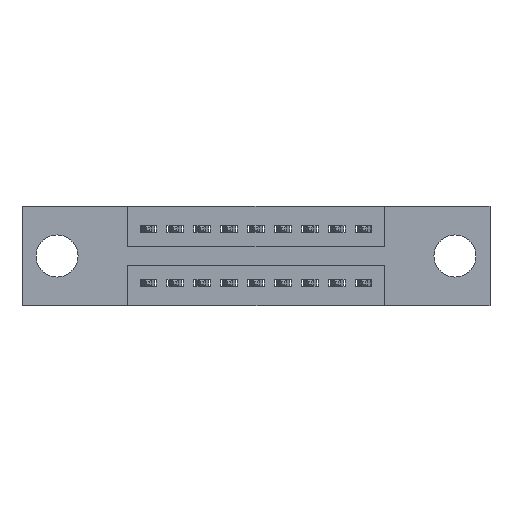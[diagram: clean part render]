
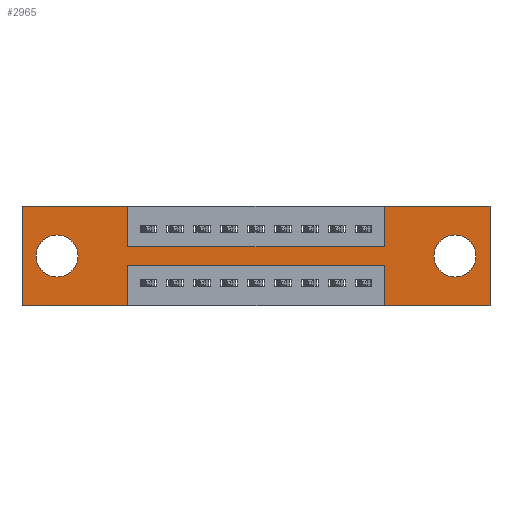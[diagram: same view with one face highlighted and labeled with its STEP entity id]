
A CAD part, front view. The second image highlights one B-rep face of the part: STEP entity #2965.
In plain terms, the highlighted planar face has unit normal (0, -1, 0).
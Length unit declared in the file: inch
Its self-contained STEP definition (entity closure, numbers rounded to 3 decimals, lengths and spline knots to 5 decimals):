
#74 = VERTEX_POINT ( 'NONE', #2329 ) ;
#160 = DIRECTION ( 'NONE',  ( 0., 0., 1. ) ) ;
#163 = VERTEX_POINT ( 'NONE', #8953 ) ;
#263 = DIRECTION ( 'NONE',  ( 0., 1., 0. ) ) ;
#372 = ORIENTED_EDGE ( 'NONE', *, *, #6283, .F. ) ;
#404 = ORIENTED_EDGE ( 'NONE', *, *, #4844, .F. ) ;
#423 = VERTEX_POINT ( 'NONE', #2195 ) ;
#517 = LINE ( 'NONE', #7329, #3308 ) ;
#692 = FACE_BOUND ( 'NONE', #3170, .T. ) ;
#868 = CARTESIAN_POINT ( 'NONE',  ( 0.3925, 0., -0.22 ) ) ;
#878 = PLANE ( 'NONE',  #1869 ) ;
#967 = VERTEX_POINT ( 'NONE', #7991 ) ;
#1048 = DIRECTION ( 'NONE',  ( 0., -1., 0. ) ) ;
#1077 = CARTESIAN_POINT ( 'NONE',  ( 1.3425, 0., 0. ) ) ;
#1246 = LINE ( 'NONE', #7580, #3026 ) ;
#1304 = ORIENTED_EDGE ( 'NONE', *, *, #8334, .T. ) ;
#1322 = ORIENTED_EDGE ( 'NONE', *, *, #5322, .T. ) ;
#1618 = DIRECTION ( 'NONE',  ( 0., 1., 0. ) ) ;
#1650 = ORIENTED_EDGE ( 'NONE', *, *, #9314, .F. ) ;
#1763 = CARTESIAN_POINT ( 'NONE',  ( 1.605, 0., -0.107 ) ) ;
#1867 = ORIENTED_EDGE ( 'NONE', *, *, #5052, .F. ) ;
#1869 = AXIS2_PLACEMENT_3D ( 'NONE', #3627, #1048, #10817 ) ;
#1968 = ORIENTED_EDGE ( 'NONE', *, *, #8434, .F. ) ;
#2028 = EDGE_CURVE ( 'NONE', #74, #2369, #5194, .T. ) ;
#2097 = VECTOR ( 'NONE', #3045, 39.37008 ) ;
#2189 = LINE ( 'NONE', #2750, #8909 ) ;
#2195 = CARTESIAN_POINT ( 'NONE',  ( 0.3925, 0., -0.15 ) ) ;
#2329 = CARTESIAN_POINT ( 'NONE',  ( 1.3425, 0., -0.22 ) ) ;
#2369 = VERTEX_POINT ( 'NONE', #9668 ) ;
#2477 = VERTEX_POINT ( 'NONE', #9061 ) ;
#2519 = VECTOR ( 'NONE', #4711, 39.37008 ) ;
#2556 = EDGE_CURVE ( 'NONE', #2369, #6684, #2641, .T. ) ;
#2635 = CARTESIAN_POINT ( 'NONE',  ( 1.605, 0., -0.185 ) ) ;
#2641 = LINE ( 'NONE', #6640, #2097 ) ;
#2654 = CARTESIAN_POINT ( 'NONE',  ( 0.3925, 0., -0.37 ) ) ;
#2666 = DIRECTION ( 'NONE',  ( 0., 1., 0. ) ) ;
#2750 = CARTESIAN_POINT ( 'NONE',  ( 0., 0., -0.37 ) ) ;
#2965 = ADVANCED_FACE ( 'NONE', ( #8938, #692, #6413 ), #878, .T. ) ;
#2986 = VERTEX_POINT ( 'NONE', #4615 ) ;
#3002 = CARTESIAN_POINT ( 'NONE',  ( 1.735, 0., 0. ) ) ;
#3004 = VECTOR ( 'NONE', #5814, 39.37008 ) ;
#3006 = CARTESIAN_POINT ( 'NONE',  ( 1.605, 0., -0.185 ) ) ;
#3026 = VECTOR ( 'NONE', #6043, 39.37008 ) ;
#3045 = DIRECTION ( 'NONE',  ( 0., 0., -1. ) ) ;
#3170 = EDGE_LOOP ( 'NONE', ( #1304, #4681 ) ) ;
#3264 = CARTESIAN_POINT ( 'NONE',  ( 0.13, 0., -0.185 ) ) ;
#3308 = VECTOR ( 'NONE', #6284, 39.37008 ) ;
#3390 = VECTOR ( 'NONE', #3605, 39.37008 ) ;
#3605 = DIRECTION ( 'NONE',  ( 0., 0., 1. ) ) ;
#3627 = CARTESIAN_POINT ( 'NONE',  ( 0., 0., -0.37 ) ) ;
#3881 = CIRCLE ( 'NONE', #6200, 0.078 ) ;
#4049 = CARTESIAN_POINT ( 'NONE',  ( 0.3925, 0., -0.15 ) ) ;
#4346 = VECTOR ( 'NONE', #9405, 39.37008 ) ;
#4452 = EDGE_CURVE ( 'NONE', #4661, #2986, #517, .T. ) ;
#4464 = VERTEX_POINT ( 'NONE', #10006 ) ;
#4508 = CARTESIAN_POINT ( 'NONE',  ( 1.3425, 0., -0.15 ) ) ;
#4511 = AXIS2_PLACEMENT_3D ( 'NONE', #3264, #1618, #9648 ) ;
#4615 = CARTESIAN_POINT ( 'NONE',  ( 0.3925, 0., 0. ) ) ;
#4624 = CARTESIAN_POINT ( 'NONE',  ( 0.3925, 0., 0. ) ) ;
#4626 = ORIENTED_EDGE ( 'NONE', *, *, #6876, .F. ) ;
#4661 = VERTEX_POINT ( 'NONE', #5817 ) ;
#4681 = ORIENTED_EDGE ( 'NONE', *, *, #5490, .T. ) ;
#4711 = DIRECTION ( 'NONE',  ( 1., 0., 0. ) ) ;
#4726 = AXIS2_PLACEMENT_3D ( 'NONE', #2635, #2666, #11544 ) ;
#4732 = EDGE_CURVE ( 'NONE', #2477, #4661, #1246, .T. ) ;
#4757 = LINE ( 'NONE', #6350, #2519 ) ;
#4844 = EDGE_CURVE ( 'NONE', #8877, #6912, #10434, .T. ) ;
#4965 = ORIENTED_EDGE ( 'NONE', *, *, #2556, .F. ) ;
#5052 = EDGE_CURVE ( 'NONE', #6912, #5566, #2189, .T. ) ;
#5060 = VECTOR ( 'NONE', #160, 39.37008 ) ;
#5194 = LINE ( 'NONE', #868, #9117 ) ;
#5232 = DIRECTION ( 'NONE',  ( 0., 0., -1. ) ) ;
#5322 = EDGE_CURVE ( 'NONE', #8414, #163, #5557, .T. ) ;
#5490 = EDGE_CURVE ( 'NONE', #6896, #967, #7483, .T. ) ;
#5550 = VECTOR ( 'NONE', #5232, 39.37008 ) ;
#5557 = CIRCLE ( 'NONE', #4726, 0.078 ) ;
#5566 = VERTEX_POINT ( 'NONE', #6068 ) ;
#5814 = DIRECTION ( 'NONE',  ( 1., 0., 0. ) ) ;
#5817 = CARTESIAN_POINT ( 'NONE',  ( 0., 0., 0. ) ) ;
#5885 = ORIENTED_EDGE ( 'NONE', *, *, #11150, .T. ) ;
#5895 = CARTESIAN_POINT ( 'NONE',  ( 0., 0., -0.37 ) ) ;
#6043 = DIRECTION ( 'NONE',  ( 0., 0., 1. ) ) ;
#6055 = EDGE_CURVE ( 'NONE', #423, #10147, #11526, .T. ) ;
#6068 = CARTESIAN_POINT ( 'NONE',  ( 1.3425, 0., -0.37 ) ) ;
#6154 = EDGE_LOOP ( 'NONE', ( #1322, #5885 ) ) ;
#6200 = AXIS2_PLACEMENT_3D ( 'NONE', #3006, #263, #9274 ) ;
#6215 = DIRECTION ( 'NONE',  ( 0., 1., 0. ) ) ;
#6283 = EDGE_CURVE ( 'NONE', #2986, #423, #11244, .T. ) ;
#6284 = DIRECTION ( 'NONE',  ( 1., 0., 0. ) ) ;
#6314 = CIRCLE ( 'NONE', #4511, 0.078 ) ;
#6346 = DIRECTION ( 'NONE',  ( -1., 0., 0. ) ) ;
#6350 = CARTESIAN_POINT ( 'NONE',  ( 0., 0., 0. ) ) ;
#6413 = FACE_OUTER_BOUND ( 'NONE', #11055, .T. ) ;
#6502 = ORIENTED_EDGE ( 'NONE', *, *, #4732, .F. ) ;
#6640 = CARTESIAN_POINT ( 'NONE',  ( 0.3925, 0., -0.37 ) ) ;
#6684 = VERTEX_POINT ( 'NONE', #2654 ) ;
#6856 = DIRECTION ( 'NONE',  ( 0., 0., -1. ) ) ;
#6876 = EDGE_CURVE ( 'NONE', #5566, #74, #6904, .T. ) ;
#6896 = VERTEX_POINT ( 'NONE', #9437 ) ;
#6904 = LINE ( 'NONE', #11414, #3390 ) ;
#6912 = VERTEX_POINT ( 'NONE', #8228 ) ;
#7075 = VECTOR ( 'NONE', #6856, 39.37008 ) ;
#7215 = ORIENTED_EDGE ( 'NONE', *, *, #8999, .F. ) ;
#7329 = CARTESIAN_POINT ( 'NONE',  ( 0., 0., 0. ) ) ;
#7483 = CIRCLE ( 'NONE', #9961, 0.078 ) ;
#7580 = CARTESIAN_POINT ( 'NONE',  ( 0., 0., 0. ) ) ;
#7991 = CARTESIAN_POINT ( 'NONE',  ( 0.13, 0., -0.107 ) ) ;
#8228 = CARTESIAN_POINT ( 'NONE',  ( 1.735, 0., -0.37 ) ) ;
#8334 = EDGE_CURVE ( 'NONE', #967, #6896, #6314, .T. ) ;
#8414 = VERTEX_POINT ( 'NONE', #1763 ) ;
#8434 = EDGE_CURVE ( 'NONE', #10147, #4464, #9802, .T. ) ;
#8478 = ORIENTED_EDGE ( 'NONE', *, *, #6055, .F. ) ;
#8682 = ORIENTED_EDGE ( 'NONE', *, *, #2028, .F. ) ;
#8877 = VERTEX_POINT ( 'NONE', #3002 ) ;
#8909 = VECTOR ( 'NONE', #6346, 39.37008 ) ;
#8938 = FACE_BOUND ( 'NONE', #6154, .T. ) ;
#8953 = CARTESIAN_POINT ( 'NONE',  ( 1.605, 0., -0.263 ) ) ;
#8999 = EDGE_CURVE ( 'NONE', #6684, #2477, #11459, .T. ) ;
#9002 = ORIENTED_EDGE ( 'NONE', *, *, #4452, .F. ) ;
#9061 = CARTESIAN_POINT ( 'NONE',  ( 0., 0., -0.37 ) ) ;
#9117 = VECTOR ( 'NONE', #11534, 39.37008 ) ;
#9274 = DIRECTION ( 'NONE',  ( 0., 0., -1. ) ) ;
#9314 = EDGE_CURVE ( 'NONE', #4464, #8877, #4757, .T. ) ;
#9405 = DIRECTION ( 'NONE',  ( -1., 0., 0. ) ) ;
#9437 = CARTESIAN_POINT ( 'NONE',  ( 0.13, 0., -0.263 ) ) ;
#9648 = DIRECTION ( 'NONE',  ( 0., 0., 1. ) ) ;
#9668 = CARTESIAN_POINT ( 'NONE',  ( 0.3925, 0., -0.22 ) ) ;
#9672 = CARTESIAN_POINT ( 'NONE',  ( 1.735, 0., 0. ) ) ;
#9801 = CARTESIAN_POINT ( 'NONE',  ( 0.13, 0., -0.185 ) ) ;
#9802 = LINE ( 'NONE', #1077, #5060 ) ;
#9961 = AXIS2_PLACEMENT_3D ( 'NONE', #9801, #6215, #11444 ) ;
#10006 = CARTESIAN_POINT ( 'NONE',  ( 1.3425, 0., 0. ) ) ;
#10147 = VERTEX_POINT ( 'NONE', #4508 ) ;
#10434 = LINE ( 'NONE', #9672, #7075 ) ;
#10817 = DIRECTION ( 'NONE',  ( 0., 0., -1. ) ) ;
#11055 = EDGE_LOOP ( 'NONE', ( #4965, #8682, #4626, #1867, #404, #1650, #1968, #8478, #372, #9002, #6502, #7215 ) ) ;
#11150 = EDGE_CURVE ( 'NONE', #163, #8414, #3881, .T. ) ;
#11244 = LINE ( 'NONE', #4624, #5550 ) ;
#11414 = CARTESIAN_POINT ( 'NONE',  ( 1.3425, 0., -0.37 ) ) ;
#11444 = DIRECTION ( 'NONE',  ( 0., 0., 1. ) ) ;
#11459 = LINE ( 'NONE', #5895, #4346 ) ;
#11526 = LINE ( 'NONE', #4049, #3004 ) ;
#11534 = DIRECTION ( 'NONE',  ( -1., 0., 0. ) ) ;
#11544 = DIRECTION ( 'NONE',  ( 0., 0., -1. ) ) ;
